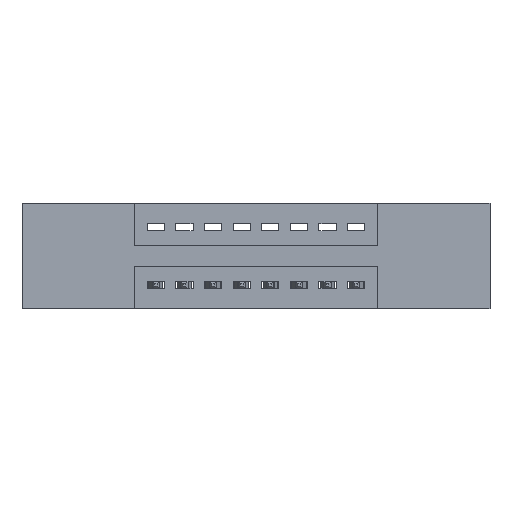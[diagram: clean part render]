
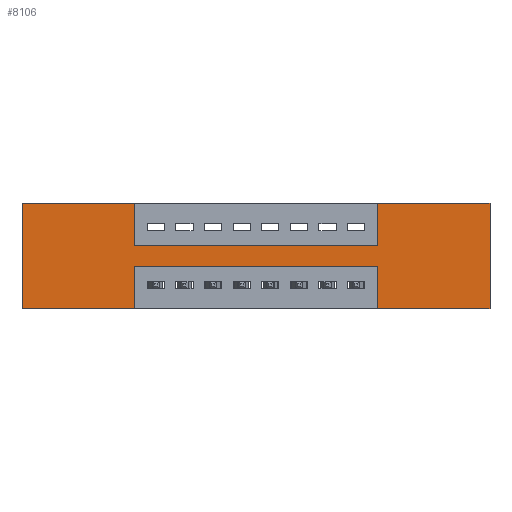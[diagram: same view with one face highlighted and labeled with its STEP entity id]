
A CAD part, front view. The second image highlights one B-rep face of the part: STEP entity #8106.
In plain terms, the highlighted planar face has unit normal (0, -1, 0).
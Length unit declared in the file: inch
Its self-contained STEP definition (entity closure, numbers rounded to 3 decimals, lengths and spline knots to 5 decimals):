
#79 = VECTOR ( 'NONE', #1190, 39.37008 ) ;
#114 = EDGE_CURVE ( 'NONE', #1149, #7425, #2945, .T. ) ;
#312 = FACE_OUTER_BOUND ( 'NONE', #7814, .T. ) ;
#345 = CARTESIAN_POINT ( 'NONE',  ( 1.2425, 0., 0. ) ) ;
#493 = EDGE_CURVE ( 'NONE', #9545, #1149, #8202, .T. ) ;
#584 = VECTOR ( 'NONE', #7531, 39.37008 ) ;
#664 = ORIENTED_EDGE ( 'NONE', *, *, #7783, .F. ) ;
#768 = CARTESIAN_POINT ( 'NONE',  ( 1.635, 0., -0.37 ) ) ;
#774 = ORIENTED_EDGE ( 'NONE', *, *, #3262, .F. ) ;
#784 = CARTESIAN_POINT ( 'NONE',  ( 0., 0., -0.37 ) ) ;
#979 = VECTOR ( 'NONE', #6738, 39.37008 ) ;
#1003 = EDGE_CURVE ( 'NONE', #9985, #5042, #3055, .T. ) ;
#1026 = VERTEX_POINT ( 'NONE', #10268 ) ;
#1149 = VERTEX_POINT ( 'NONE', #8805 ) ;
#1170 = DIRECTION ( 'NONE',  ( 0., 0., 1. ) ) ;
#1186 = VERTEX_POINT ( 'NONE', #4807 ) ;
#1190 = DIRECTION ( 'NONE',  ( 0., 0., -1. ) ) ;
#1323 = DIRECTION ( 'NONE',  ( 0., -1., 0. ) ) ;
#1400 = DIRECTION ( 'NONE',  ( 0., 0., -1. ) ) ;
#1590 = ORIENTED_EDGE ( 'NONE', *, *, #9256, .F. ) ;
#2049 = CARTESIAN_POINT ( 'NONE',  ( 0., 0., -0.37 ) ) ;
#2117 = LINE ( 'NONE', #5287, #7034 ) ;
#2330 = VERTEX_POINT ( 'NONE', #3005 ) ;
#2395 = ORIENTED_EDGE ( 'NONE', *, *, #6821, .F. ) ;
#2632 = DIRECTION ( 'NONE',  ( 1., 0., 0. ) ) ;
#2673 = EDGE_CURVE ( 'NONE', #3298, #9545, #9715, .T. ) ;
#2945 = LINE ( 'NONE', #5290, #4241 ) ;
#2992 = DIRECTION ( 'NONE',  ( 1., 0., 0. ) ) ;
#3005 = CARTESIAN_POINT ( 'NONE',  ( 0., 0., -0.37 ) ) ;
#3055 = LINE ( 'NONE', #8617, #5257 ) ;
#3095 = ORIENTED_EDGE ( 'NONE', *, *, #4668, .F. ) ;
#3262 = EDGE_CURVE ( 'NONE', #7912, #7523, #5844, .T. ) ;
#3298 = VERTEX_POINT ( 'NONE', #8494 ) ;
#3494 = CARTESIAN_POINT ( 'NONE',  ( 0.3925, 0., -0.37 ) ) ;
#3553 = CARTESIAN_POINT ( 'NONE',  ( 0.3925, 0., -0.37 ) ) ;
#3675 = PLANE ( 'NONE',  #7816 ) ;
#4226 = CARTESIAN_POINT ( 'NONE',  ( 0.3925, 0., -0.15 ) ) ;
#4231 = LINE ( 'NONE', #5919, #6676 ) ;
#4241 = VECTOR ( 'NONE', #7729, 39.37008 ) ;
#4281 = CARTESIAN_POINT ( 'NONE',  ( 1.2425, 0., -0.22 ) ) ;
#4355 = CARTESIAN_POINT ( 'NONE',  ( 0.3925, 0., -0.22 ) ) ;
#4668 = EDGE_CURVE ( 'NONE', #2330, #9985, #4231, .T. ) ;
#4751 = CARTESIAN_POINT ( 'NONE',  ( 0., 0., 0. ) ) ;
#4807 = CARTESIAN_POINT ( 'NONE',  ( 1.2425, 0., -0.37 ) ) ;
#4968 = LINE ( 'NONE', #784, #8016 ) ;
#4979 = VECTOR ( 'NONE', #2632, 39.37008 ) ;
#5042 = VERTEX_POINT ( 'NONE', #8922 ) ;
#5173 = CARTESIAN_POINT ( 'NONE',  ( 1.2425, 0., 0. ) ) ;
#5257 = VECTOR ( 'NONE', #2992, 39.37008 ) ;
#5287 = CARTESIAN_POINT ( 'NONE',  ( 1.2425, 0., -0.37 ) ) ;
#5290 = CARTESIAN_POINT ( 'NONE',  ( 1.635, 0., 0. ) ) ;
#5478 = LINE ( 'NONE', #3494, #584 ) ;
#5500 = DIRECTION ( 'NONE',  ( 1., 0., 0. ) ) ;
#5529 = VECTOR ( 'NONE', #5500, 39.37008 ) ;
#5542 = CARTESIAN_POINT ( 'NONE',  ( 0., 0., -0.37 ) ) ;
#5777 = ORIENTED_EDGE ( 'NONE', *, *, #1003, .F. ) ;
#5844 = LINE ( 'NONE', #4355, #6930 ) ;
#5919 = CARTESIAN_POINT ( 'NONE',  ( 0., 0., 0. ) ) ;
#6068 = VERTEX_POINT ( 'NONE', #3553 ) ;
#6268 = CARTESIAN_POINT ( 'NONE',  ( 0.3925, 0., -0.22 ) ) ;
#6496 = LINE ( 'NONE', #9913, #79 ) ;
#6588 = CARTESIAN_POINT ( 'NONE',  ( 0., 0., 0. ) ) ;
#6676 = VECTOR ( 'NONE', #9944, 39.37008 ) ;
#6738 = DIRECTION ( 'NONE',  ( 0., 0., 1. ) ) ;
#6779 = ORIENTED_EDGE ( 'NONE', *, *, #7049, .F. ) ;
#6820 = ORIENTED_EDGE ( 'NONE', *, *, #10510, .F. ) ;
#6821 = EDGE_CURVE ( 'NONE', #5042, #1026, #6496, .T. ) ;
#6930 = VECTOR ( 'NONE', #10080, 39.37008 ) ;
#7034 = VECTOR ( 'NONE', #1170, 39.37008 ) ;
#7049 = EDGE_CURVE ( 'NONE', #1026, #3298, #10341, .T. ) ;
#7425 = VERTEX_POINT ( 'NONE', #768 ) ;
#7523 = VERTEX_POINT ( 'NONE', #6268 ) ;
#7531 = DIRECTION ( 'NONE',  ( 0., 0., -1. ) ) ;
#7729 = DIRECTION ( 'NONE',  ( 0., 0., -1. ) ) ;
#7773 = VECTOR ( 'NONE', #7942, 39.37008 ) ;
#7783 = EDGE_CURVE ( 'NONE', #7425, #1186, #4968, .T. ) ;
#7814 = EDGE_LOOP ( 'NONE', ( #6820, #774, #1590, #664, #8551, #8953, #9499, #6779, #2395, #5777, #3095, #8469 ) ) ;
#7816 = AXIS2_PLACEMENT_3D ( 'NONE', #2049, #1323, #1400 ) ;
#7912 = VERTEX_POINT ( 'NONE', #4281 ) ;
#7942 = DIRECTION ( 'NONE',  ( -1., 0., 0. ) ) ;
#8016 = VECTOR ( 'NONE', #9841, 39.37008 ) ;
#8106 = ADVANCED_FACE ( 'NONE', ( #312 ), #3675, .T. ) ;
#8153 = EDGE_CURVE ( 'NONE', #6068, #2330, #8262, .T. ) ;
#8202 = LINE ( 'NONE', #4751, #5529 ) ;
#8262 = LINE ( 'NONE', #5542, #7773 ) ;
#8469 = ORIENTED_EDGE ( 'NONE', *, *, #8153, .F. ) ;
#8494 = CARTESIAN_POINT ( 'NONE',  ( 1.2425, 0., -0.15 ) ) ;
#8551 = ORIENTED_EDGE ( 'NONE', *, *, #114, .F. ) ;
#8617 = CARTESIAN_POINT ( 'NONE',  ( 0., 0., 0. ) ) ;
#8805 = CARTESIAN_POINT ( 'NONE',  ( 1.635, 0., 0. ) ) ;
#8922 = CARTESIAN_POINT ( 'NONE',  ( 0.3925, 0., 0. ) ) ;
#8953 = ORIENTED_EDGE ( 'NONE', *, *, #493, .F. ) ;
#9256 = EDGE_CURVE ( 'NONE', #1186, #7912, #2117, .T. ) ;
#9499 = ORIENTED_EDGE ( 'NONE', *, *, #2673, .F. ) ;
#9545 = VERTEX_POINT ( 'NONE', #345 ) ;
#9715 = LINE ( 'NONE', #5173, #979 ) ;
#9841 = DIRECTION ( 'NONE',  ( -1., 0., 0. ) ) ;
#9913 = CARTESIAN_POINT ( 'NONE',  ( 0.3925, 0., 0. ) ) ;
#9944 = DIRECTION ( 'NONE',  ( 0., 0., 1. ) ) ;
#9985 = VERTEX_POINT ( 'NONE', #6588 ) ;
#10080 = DIRECTION ( 'NONE',  ( -1., 0., 0. ) ) ;
#10268 = CARTESIAN_POINT ( 'NONE',  ( 0.3925, 0., -0.15 ) ) ;
#10341 = LINE ( 'NONE', #4226, #4979 ) ;
#10510 = EDGE_CURVE ( 'NONE', #7523, #6068, #5478, .T. ) ;
